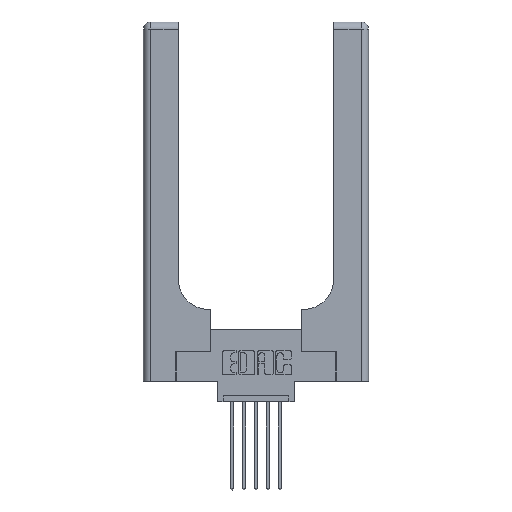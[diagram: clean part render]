
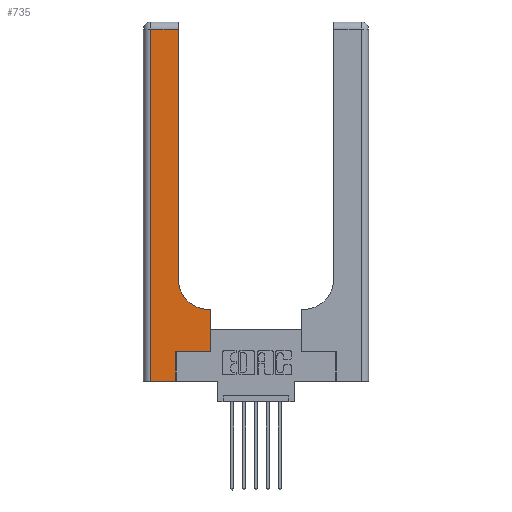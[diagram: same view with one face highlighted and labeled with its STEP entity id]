
A CAD part, top view. The second image highlights one B-rep face of the part: STEP entity #735.
In plain terms, the highlighted planar face has unit normal (0, 0, 1).
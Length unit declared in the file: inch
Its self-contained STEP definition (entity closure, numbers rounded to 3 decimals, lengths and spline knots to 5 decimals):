
#157 = CARTESIAN_POINT ( 'NONE',  ( 0.269, 0., 0.37 ) ) ;
#575 = VERTEX_POINT ( 'NONE', #1450 ) ;
#735 = ADVANCED_FACE ( 'NONE', ( #5330 ), #12294, .F. ) ;
#938 = CARTESIAN_POINT ( 'NONE',  ( 0.269, 0.25, 0.37 ) ) ;
#1169 = DIRECTION ( 'NONE',  ( 1., 0., 0. ) ) ;
#1450 = CARTESIAN_POINT ( 'NONE',  ( 0.5415, 0.6, 0.37 ) ) ;
#1474 = DIRECTION ( 'NONE',  ( 0., 0., -1. ) ) ;
#1614 = VECTOR ( 'NONE', #9540, 39.37008 ) ;
#1673 = CARTESIAN_POINT ( 'NONE',  ( 0.269, 0., 0.37 ) ) ;
#1798 = VERTEX_POINT ( 'NONE', #938 ) ;
#1824 = ORIENTED_EDGE ( 'NONE', *, *, #7499, .T. ) ;
#1991 = VERTEX_POINT ( 'NONE', #10733 ) ;
#2096 = CARTESIAN_POINT ( 'NONE',  ( 0.5585, 0.25, 0.37 ) ) ;
#2250 = DIRECTION ( 'NONE',  ( 1., 0., 0. ) ) ;
#2346 = LINE ( 'NONE', #6710, #2684 ) ;
#2426 = CARTESIAN_POINT ( 'NONE',  ( 0., 3., 0.37 ) ) ;
#2684 = VECTOR ( 'NONE', #3425, 39.37008 ) ;
#3425 = DIRECTION ( 'NONE',  ( -1., 0., 0. ) ) ;
#3579 = VERTEX_POINT ( 'NONE', #6684 ) ;
#3606 = ORIENTED_EDGE ( 'NONE', *, *, #11448, .T. ) ;
#3730 = CARTESIAN_POINT ( 'NONE',  ( 0.5415, 0.85, 0.37 ) ) ;
#3779 = DIRECTION ( 'NONE',  ( 0., 0., -1. ) ) ;
#3828 = DIRECTION ( 'NONE',  ( 1., 0., 0. ) ) ;
#4330 = LINE ( 'NONE', #6332, #1614 ) ;
#4675 = VERTEX_POINT ( 'NONE', #157 ) ;
#4706 = EDGE_LOOP ( 'NONE', ( #13243, #7209, #11336, #11615, #3606, #1824, #12637, #7305, #7155 ) ) ;
#4795 = DIRECTION ( 'NONE',  ( 0., 1., 0. ) ) ;
#4950 = DIRECTION ( 'NONE',  ( 0., -1., 0. ) ) ;
#5026 = EDGE_CURVE ( 'NONE', #8253, #575, #12176, .T. ) ;
#5330 = FACE_OUTER_BOUND ( 'NONE', #4706, .T. ) ;
#5485 = VECTOR ( 'NONE', #2250, 39.37008 ) ;
#5534 = VECTOR ( 'NONE', #1169, 39.37008 ) ;
#5571 = CARTESIAN_POINT ( 'NONE',  ( 0.269, 0.25, 0.37 ) ) ;
#5815 = CARTESIAN_POINT ( 'NONE',  ( 0.06, 0., 0.37 ) ) ;
#6332 = CARTESIAN_POINT ( 'NONE',  ( 0.2915, 3., 0.37 ) ) ;
#6352 = EDGE_CURVE ( 'NONE', #3579, #1991, #2346, .T. ) ;
#6428 = CIRCLE ( 'NONE', #7636, 0.25 ) ;
#6611 = CARTESIAN_POINT ( 'NONE',  ( 0.2915, 0.6, 0.37 ) ) ;
#6684 = CARTESIAN_POINT ( 'NONE',  ( 0.2915, 2.94, 0.37 ) ) ;
#6710 = CARTESIAN_POINT ( 'NONE',  ( 0., 2.94, 0.37 ) ) ;
#7155 = ORIENTED_EDGE ( 'NONE', *, *, #11877, .T. ) ;
#7158 = VERTEX_POINT ( 'NONE', #5815 ) ;
#7209 = ORIENTED_EDGE ( 'NONE', *, *, #6352, .T. ) ;
#7305 = ORIENTED_EDGE ( 'NONE', *, *, #5026, .T. ) ;
#7344 = EDGE_CURVE ( 'NONE', #9123, #8253, #12526, .T. ) ;
#7436 = CARTESIAN_POINT ( 'NONE',  ( 0.5585, 0.25, 0.37 ) ) ;
#7499 = EDGE_CURVE ( 'NONE', #1798, #9123, #13548, .T. ) ;
#7535 = DIRECTION ( 'NONE',  ( 0., 1., 0. ) ) ;
#7636 = AXIS2_PLACEMENT_3D ( 'NONE', #3730, #3779, #3828 ) ;
#7716 = AXIS2_PLACEMENT_3D ( 'NONE', #2426, #1474, #7873 ) ;
#7868 = EDGE_CURVE ( 'NONE', #1991, #7158, #13535, .T. ) ;
#7873 = DIRECTION ( 'NONE',  ( -1., 0., 0. ) ) ;
#8253 = VERTEX_POINT ( 'NONE', #13332 ) ;
#8369 = VERTEX_POINT ( 'NONE', #13761 ) ;
#8506 = LINE ( 'NONE', #1673, #13978 ) ;
#8528 = EDGE_CURVE ( 'NONE', #8369, #3579, #4330, .T. ) ;
#9123 = VERTEX_POINT ( 'NONE', #2096 ) ;
#9540 = DIRECTION ( 'NONE',  ( 0., 1., 0. ) ) ;
#9561 = LINE ( 'NONE', #10018, #5485 ) ;
#9627 = VECTOR ( 'NONE', #7535, 39.37008 ) ;
#9773 = VECTOR ( 'NONE', #4950, 39.37008 ) ;
#10018 = CARTESIAN_POINT ( 'NONE',  ( 0., 0., 0.37 ) ) ;
#10375 = CARTESIAN_POINT ( 'NONE',  ( 0.06, 3., 0.37 ) ) ;
#10733 = CARTESIAN_POINT ( 'NONE',  ( 0.06, 2.94, 0.37 ) ) ;
#11336 = ORIENTED_EDGE ( 'NONE', *, *, #7868, .T. ) ;
#11448 = EDGE_CURVE ( 'NONE', #4675, #1798, #8506, .T. ) ;
#11615 = ORIENTED_EDGE ( 'NONE', *, *, #12806, .T. ) ;
#11877 = EDGE_CURVE ( 'NONE', #575, #8369, #6428, .T. ) ;
#12176 = LINE ( 'NONE', #6611, #13367 ) ;
#12294 = PLANE ( 'NONE',  #7716 ) ;
#12526 = LINE ( 'NONE', #7436, #9627 ) ;
#12637 = ORIENTED_EDGE ( 'NONE', *, *, #7344, .T. ) ;
#12806 = EDGE_CURVE ( 'NONE', #7158, #4675, #9561, .T. ) ;
#13071 = DIRECTION ( 'NONE',  ( -1., 0., 0. ) ) ;
#13243 = ORIENTED_EDGE ( 'NONE', *, *, #8528, .T. ) ;
#13332 = CARTESIAN_POINT ( 'NONE',  ( 0.5585, 0.6, 0.37 ) ) ;
#13367 = VECTOR ( 'NONE', #13071, 39.37008 ) ;
#13535 = LINE ( 'NONE', #10375, #9773 ) ;
#13548 = LINE ( 'NONE', #5571, #5534 ) ;
#13761 = CARTESIAN_POINT ( 'NONE',  ( 0.2915, 0.85, 0.37 ) ) ;
#13978 = VECTOR ( 'NONE', #4795, 39.37008 ) ;
